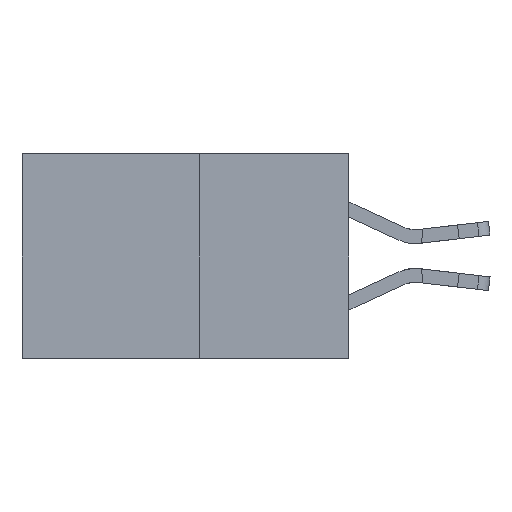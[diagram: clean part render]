
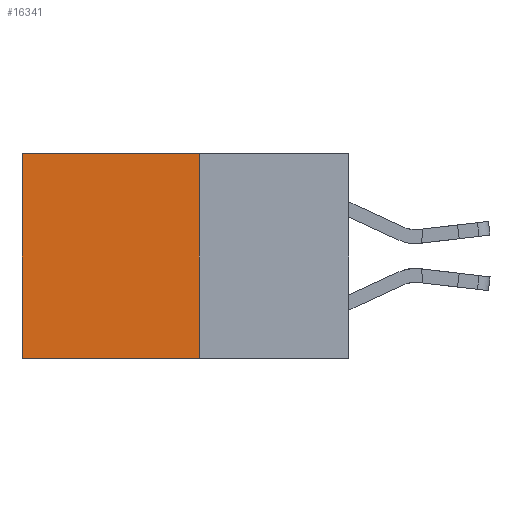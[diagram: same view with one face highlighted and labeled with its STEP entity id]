
A CAD part, left-side view. The second image highlights one B-rep face of the part: STEP entity #16341.
In plain terms, the highlighted planar face has unit normal (-1, 0, 0).
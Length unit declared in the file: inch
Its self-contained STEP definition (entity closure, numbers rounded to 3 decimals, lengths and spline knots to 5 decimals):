
#1732 = CARTESIAN_POINT ( 'NONE',  ( 0.277, 0.27, -0.37 ) ) ;
#1851 = CARTESIAN_POINT ( 'NONE',  ( 0.277, 0.59, -0.37 ) ) ;
#2207 = ORIENTED_EDGE ( 'NONE', *, *, #26616, .T. ) ;
#2635 = LINE ( 'NONE', #17438, #14152 ) ;
#2846 = VECTOR ( 'NONE', #19314, 39.37008 ) ;
#3384 = CARTESIAN_POINT ( 'NONE',  ( 0.277, 0.59, -0.37 ) ) ;
#3674 = EDGE_CURVE ( 'NONE', #23605, #20996, #9209, .T. ) ;
#3953 = PLANE ( 'NONE',  #13156 ) ;
#4863 = ORIENTED_EDGE ( 'NONE', *, *, #3674, .T. ) ;
#5145 = EDGE_CURVE ( 'NONE', #9003, #20996, #2635, .T. ) ;
#5216 = DIRECTION ( 'NONE',  ( 0., 0., -1. ) ) ;
#5274 = EDGE_LOOP ( 'NONE', ( #4863, #7552, #25697, #2207 ) ) ;
#5674 = VERTEX_POINT ( 'NONE', #10755 ) ;
#5768 = CARTESIAN_POINT ( 'NONE',  ( 0.277, 0.59, 0. ) ) ;
#6687 = DIRECTION ( 'NONE',  ( 0., 1., 0. ) ) ;
#7343 = VECTOR ( 'NONE', #5216, 39.37008 ) ;
#7415 = CARTESIAN_POINT ( 'NONE',  ( 0.277, 0.27, -0.37 ) ) ;
#7552 = ORIENTED_EDGE ( 'NONE', *, *, #5145, .F. ) ;
#8334 = DIRECTION ( 'NONE',  ( 1., 0., 0. ) ) ;
#9003 = VERTEX_POINT ( 'NONE', #9457 ) ;
#9209 = LINE ( 'NONE', #1851, #14933 ) ;
#9457 = CARTESIAN_POINT ( 'NONE',  ( 0.277, 0.27, -0.37 ) ) ;
#10755 = CARTESIAN_POINT ( 'NONE',  ( 0.277, 0.27, 0. ) ) ;
#11769 = DIRECTION ( 'NONE',  ( 0., 0., -1. ) ) ;
#13156 = AXIS2_PLACEMENT_3D ( 'NONE', #1732, #8334, #23367 ) ;
#14152 = VECTOR ( 'NONE', #6687, 39.37008 ) ;
#14860 = CARTESIAN_POINT ( 'NONE',  ( 0.277, 0.27, 0. ) ) ;
#14933 = VECTOR ( 'NONE', #11769, 39.37008 ) ;
#16341 = ADVANCED_FACE ( 'NONE', ( #19732 ), #3953, .F. ) ;
#17438 = CARTESIAN_POINT ( 'NONE',  ( 0.277, 0.27, -0.37 ) ) ;
#18834 = LINE ( 'NONE', #7415, #7343 ) ;
#19314 = DIRECTION ( 'NONE',  ( 0., 1., 0. ) ) ;
#19732 = FACE_OUTER_BOUND ( 'NONE', #5274, .T. ) ;
#20151 = LINE ( 'NONE', #14860, #2846 ) ;
#20477 = EDGE_CURVE ( 'NONE', #5674, #9003, #18834, .T. ) ;
#20996 = VERTEX_POINT ( 'NONE', #3384 ) ;
#23367 = DIRECTION ( 'NONE',  ( 0., 0., -1. ) ) ;
#23605 = VERTEX_POINT ( 'NONE', #5768 ) ;
#25697 = ORIENTED_EDGE ( 'NONE', *, *, #20477, .F. ) ;
#26616 = EDGE_CURVE ( 'NONE', #5674, #23605, #20151, .T. ) ;
